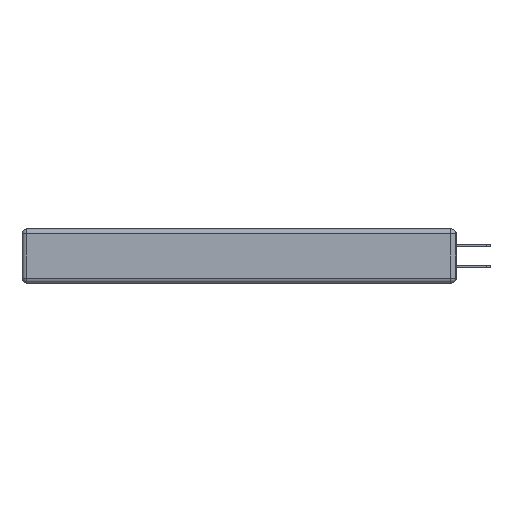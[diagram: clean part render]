
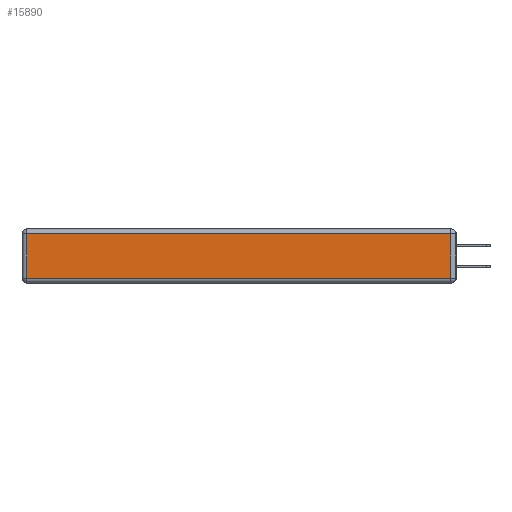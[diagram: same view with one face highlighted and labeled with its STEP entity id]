
A CAD part, left-side view. The second image highlights one B-rep face of the part: STEP entity #15890.
In plain terms, the highlighted planar face has unit normal (-1, 0, 0).
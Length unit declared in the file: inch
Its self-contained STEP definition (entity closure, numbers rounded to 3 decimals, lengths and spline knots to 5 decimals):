
#499 = VERTEX_POINT ( 'NONE', #5930 ) ;
#956 = VECTOR ( 'NONE', #14128, 39.37008 ) ;
#2278 = LINE ( 'NONE', #4275, #956 ) ;
#2402 = CARTESIAN_POINT ( 'NONE',  ( 0., 2.72, -0.313 ) ) ;
#3362 = EDGE_CURVE ( 'NONE', #4495, #499, #2278, .T. ) ;
#3411 = EDGE_CURVE ( 'NONE', #4321, #11684, #8710, .T. ) ;
#3430 = FACE_OUTER_BOUND ( 'NONE', #5197, .T. ) ;
#3604 = CARTESIAN_POINT ( 'NONE',  ( 0., 0.03, -0.343 ) ) ;
#4275 = CARTESIAN_POINT ( 'NONE',  ( 0., 0., -0.313 ) ) ;
#4321 = VERTEX_POINT ( 'NONE', #17602 ) ;
#4345 = ORIENTED_EDGE ( 'NONE', *, *, #3362, .T. ) ;
#4495 = VERTEX_POINT ( 'NONE', #2402 ) ;
#4604 = PLANE ( 'NONE',  #9129 ) ;
#4656 = CARTESIAN_POINT ( 'NONE',  ( 0., 2.72, -0.343 ) ) ;
#5165 = VECTOR ( 'NONE', #14411, 39.37008 ) ;
#5197 = EDGE_LOOP ( 'NONE', ( #4345, #9103, #11498, #15820 ) ) ;
#5913 = DIRECTION ( 'NONE',  ( 0., 0., 1. ) ) ;
#5930 = CARTESIAN_POINT ( 'NONE',  ( 0., 0.03, -0.313 ) ) ;
#6916 = LINE ( 'NONE', #4656, #5165 ) ;
#8212 = DIRECTION ( 'NONE',  ( 0., 0., 1. ) ) ;
#8710 = LINE ( 'NONE', #12810, #11805 ) ;
#9103 = ORIENTED_EDGE ( 'NONE', *, *, #13066, .T. ) ;
#9129 = AXIS2_PLACEMENT_3D ( 'NONE', #10347, #11532, #5913 ) ;
#9187 = CARTESIAN_POINT ( 'NONE',  ( 0., 2.72, -0.03 ) ) ;
#9940 = DIRECTION ( 'NONE',  ( 0., 1., 0. ) ) ;
#10347 = CARTESIAN_POINT ( 'NONE',  ( 0., 0., -0.343 ) ) ;
#10396 = EDGE_CURVE ( 'NONE', #11684, #4495, #6916, .T. ) ;
#11498 = ORIENTED_EDGE ( 'NONE', *, *, #3411, .T. ) ;
#11532 = DIRECTION ( 'NONE',  ( -1., 0., 0. ) ) ;
#11684 = VERTEX_POINT ( 'NONE', #9187 ) ;
#11805 = VECTOR ( 'NONE', #9940, 39.37008 ) ;
#12580 = VECTOR ( 'NONE', #8212, 39.37008 ) ;
#12810 = CARTESIAN_POINT ( 'NONE',  ( 0., 2.75, -0.03 ) ) ;
#13066 = EDGE_CURVE ( 'NONE', #499, #4321, #13932, .T. ) ;
#13932 = LINE ( 'NONE', #3604, #12580 ) ;
#14128 = DIRECTION ( 'NONE',  ( 0., -1., 0. ) ) ;
#14411 = DIRECTION ( 'NONE',  ( 0., 0., -1. ) ) ;
#15820 = ORIENTED_EDGE ( 'NONE', *, *, #10396, .T. ) ;
#15890 = ADVANCED_FACE ( 'NONE', ( #3430 ), #4604, .T. ) ;
#17602 = CARTESIAN_POINT ( 'NONE',  ( 0., 0.03, -0.03 ) ) ;
